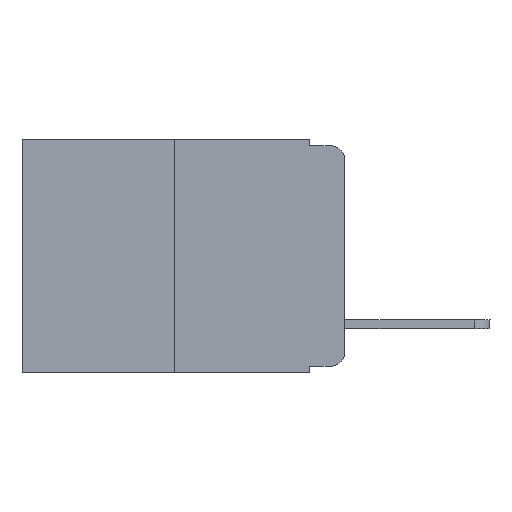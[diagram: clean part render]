
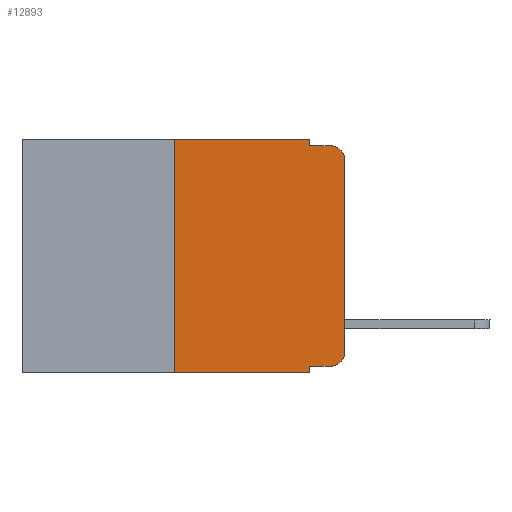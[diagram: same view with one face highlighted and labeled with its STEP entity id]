
A CAD part, left-side view. The second image highlights one B-rep face of the part: STEP entity #12893.
In plain terms, the highlighted planar face has unit normal (-1, 0, 0).
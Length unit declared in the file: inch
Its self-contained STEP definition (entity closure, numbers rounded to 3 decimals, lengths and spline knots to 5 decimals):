
#12 = ORIENTED_EDGE ( 'NONE', *, *, #9825, .T. ) ;
#30 = CARTESIAN_POINT ( 'NONE',  ( 0., 0.051, 0. ) ) ;
#243 = CARTESIAN_POINT ( 'NONE',  ( 0., 0., -0.313 ) ) ;
#299 = VERTEX_POINT ( 'NONE', #639 ) ;
#316 = LINE ( 'NONE', #12429, #13057 ) ;
#331 = ORIENTED_EDGE ( 'NONE', *, *, #11867, .T. ) ;
#544 = VECTOR ( 'NONE', #5286, 39.37008 ) ;
#580 = VECTOR ( 'NONE', #9935, 39.37008 ) ;
#639 = CARTESIAN_POINT ( 'NONE',  ( 0., 0.25, -0.343 ) ) ;
#1028 = DIRECTION ( 'NONE',  ( 0., 0., 1. ) ) ;
#1160 = EDGE_CURVE ( 'NONE', #2179, #1327, #9671, .T. ) ;
#1327 = VERTEX_POINT ( 'NONE', #7996 ) ;
#1332 = LINE ( 'NONE', #5790, #5784 ) ;
#2076 = LINE ( 'NONE', #7601, #544 ) ;
#2095 = EDGE_CURVE ( 'NONE', #10620, #7134, #5359, .T. ) ;
#2163 = VECTOR ( 'NONE', #12152, 39.37008 ) ;
#2179 = VERTEX_POINT ( 'NONE', #5648 ) ;
#2239 = CARTESIAN_POINT ( 'NONE',  ( 0., 0., -0.03 ) ) ;
#2419 = CARTESIAN_POINT ( 'NONE',  ( 0., 0.02, -0.313 ) ) ;
#2504 = CARTESIAN_POINT ( 'NONE',  ( 0., 0.051, -0.333 ) ) ;
#2516 = CIRCLE ( 'NONE', #9493, 0.02 ) ;
#2521 = CARTESIAN_POINT ( 'NONE',  ( 0., 0.02, -0.333 ) ) ;
#2678 = FACE_OUTER_BOUND ( 'NONE', #6796, .T. ) ;
#2744 = PLANE ( 'NONE',  #8595 ) ;
#3087 = ORIENTED_EDGE ( 'NONE', *, *, #3537, .T. ) ;
#3123 = ORIENTED_EDGE ( 'NONE', *, *, #2095, .F. ) ;
#3349 = VECTOR ( 'NONE', #1028, 39.37008 ) ;
#3388 = DIRECTION ( 'NONE',  ( 0., -1., 0. ) ) ;
#3490 = ORIENTED_EDGE ( 'NONE', *, *, #8209, .F. ) ;
#3537 = EDGE_CURVE ( 'NONE', #12652, #3669, #10183, .T. ) ;
#3669 = VERTEX_POINT ( 'NONE', #4657 ) ;
#4082 = CARTESIAN_POINT ( 'NONE',  ( 0., 0.02, -0.03 ) ) ;
#4514 = DIRECTION ( 'NONE',  ( -1., 0., 0. ) ) ;
#4657 = CARTESIAN_POINT ( 'NONE',  ( 0., 0.02, -0.01 ) ) ;
#5005 = DIRECTION ( 'NONE',  ( 1., 0., 0. ) ) ;
#5286 = DIRECTION ( 'NONE',  ( 0., -1., 0. ) ) ;
#5294 = CARTESIAN_POINT ( 'NONE',  ( 0., 0., 0. ) ) ;
#5359 = LINE ( 'NONE', #30, #2163 ) ;
#5541 = CARTESIAN_POINT ( 'NONE',  ( 0., 0.051, -0.343 ) ) ;
#5648 = CARTESIAN_POINT ( 'NONE',  ( 0., 0.051, 0. ) ) ;
#5758 = CARTESIAN_POINT ( 'NONE',  ( 0., 0.473, 0. ) ) ;
#5784 = VECTOR ( 'NONE', #3388, 39.37008 ) ;
#5790 = CARTESIAN_POINT ( 'NONE',  ( 0., 0.051, -0.01 ) ) ;
#6414 = DIRECTION ( 'NONE',  ( 0., 0., -1. ) ) ;
#6428 = ORIENTED_EDGE ( 'NONE', *, *, #1160, .F. ) ;
#6564 = LINE ( 'NONE', #10986, #3349 ) ;
#6796 = EDGE_LOOP ( 'NONE', ( #10614, #3087, #3490, #6428, #8081, #12067, #12, #3123, #11139, #331 ) ) ;
#6799 = VECTOR ( 'NONE', #10323, 39.37008 ) ;
#7009 = DIRECTION ( 'NONE',  ( 0., 0., -1. ) ) ;
#7112 = CARTESIAN_POINT ( 'NONE',  ( 0., 0.473, 0. ) ) ;
#7134 = VERTEX_POINT ( 'NONE', #5541 ) ;
#7258 = DIRECTION ( 'NONE',  ( 0., 0., -1. ) ) ;
#7375 = CARTESIAN_POINT ( 'NONE',  ( 0., 0.25, 0. ) ) ;
#7601 = CARTESIAN_POINT ( 'NONE',  ( 0., 0.051, -0.333 ) ) ;
#7996 = CARTESIAN_POINT ( 'NONE',  ( 0., 0.051, -0.01 ) ) ;
#8081 = ORIENTED_EDGE ( 'NONE', *, *, #8634, .F. ) ;
#8209 = EDGE_CURVE ( 'NONE', #1327, #3669, #1332, .T. ) ;
#8595 = AXIS2_PLACEMENT_3D ( 'NONE', #7112, #5005, #7258 ) ;
#8634 = EDGE_CURVE ( 'NONE', #11631, #2179, #12626, .T. ) ;
#9024 = VERTEX_POINT ( 'NONE', #2521 ) ;
#9044 = DIRECTION ( 'NONE',  ( -1., 0., 0. ) ) ;
#9226 = EDGE_CURVE ( 'NONE', #10620, #9024, #2076, .T. ) ;
#9493 = AXIS2_PLACEMENT_3D ( 'NONE', #2419, #9044, #7009 ) ;
#9671 = LINE ( 'NONE', #14088, #10046 ) ;
#9825 = EDGE_CURVE ( 'NONE', #299, #7134, #316, .T. ) ;
#9935 = DIRECTION ( 'NONE',  ( 0., 0., 1. ) ) ;
#10046 = VECTOR ( 'NONE', #6414, 39.37008 ) ;
#10122 = EDGE_CURVE ( 'NONE', #299, #11631, #6564, .T. ) ;
#10183 = CIRCLE ( 'NONE', #12016, 0.02 ) ;
#10323 = DIRECTION ( 'NONE',  ( 0., -1., 0. ) ) ;
#10614 = ORIENTED_EDGE ( 'NONE', *, *, #14257, .T. ) ;
#10620 = VERTEX_POINT ( 'NONE', #2504 ) ;
#10986 = CARTESIAN_POINT ( 'NONE',  ( 0., 0.25, 0. ) ) ;
#11139 = ORIENTED_EDGE ( 'NONE', *, *, #9226, .T. ) ;
#11631 = VERTEX_POINT ( 'NONE', #7375 ) ;
#11867 = EDGE_CURVE ( 'NONE', #9024, #11955, #2516, .T. ) ;
#11955 = VERTEX_POINT ( 'NONE', #243 ) ;
#12016 = AXIS2_PLACEMENT_3D ( 'NONE', #4082, #4514, #13359 ) ;
#12067 = ORIENTED_EDGE ( 'NONE', *, *, #10122, .F. ) ;
#12152 = DIRECTION ( 'NONE',  ( 0., 0., -1. ) ) ;
#12166 = LINE ( 'NONE', #5294, #580 ) ;
#12359 = DIRECTION ( 'NONE',  ( 0., -1., 0. ) ) ;
#12429 = CARTESIAN_POINT ( 'NONE',  ( 0., 0.473, -0.343 ) ) ;
#12626 = LINE ( 'NONE', #5758, #6799 ) ;
#12652 = VERTEX_POINT ( 'NONE', #2239 ) ;
#12893 = ADVANCED_FACE ( 'NONE', ( #2678 ), #2744, .F. ) ;
#13057 = VECTOR ( 'NONE', #12359, 39.37008 ) ;
#13359 = DIRECTION ( 'NONE',  ( 0., 0., -1. ) ) ;
#14088 = CARTESIAN_POINT ( 'NONE',  ( 0., 0.051, 0. ) ) ;
#14257 = EDGE_CURVE ( 'NONE', #11955, #12652, #12166, .T. ) ;
